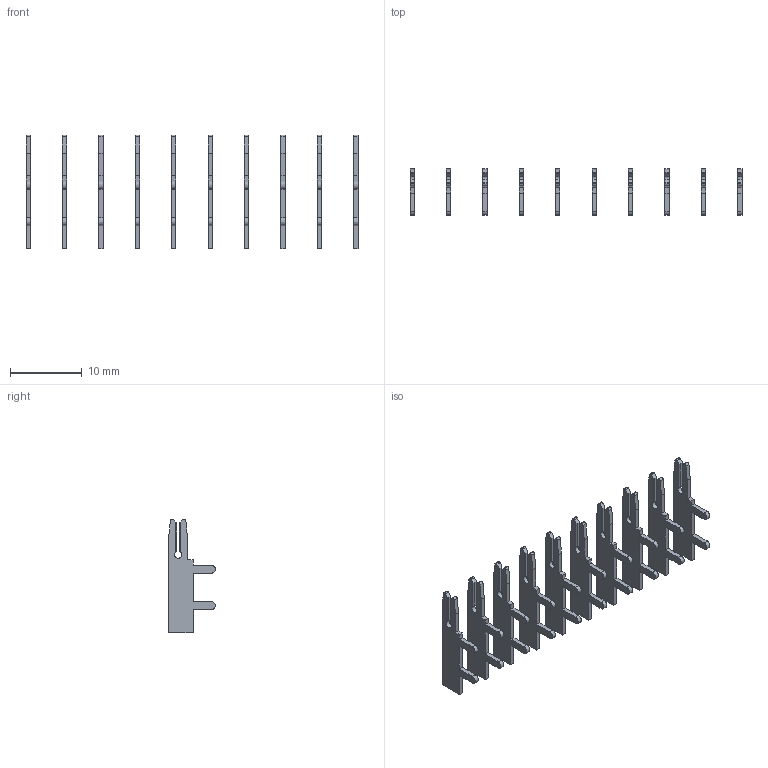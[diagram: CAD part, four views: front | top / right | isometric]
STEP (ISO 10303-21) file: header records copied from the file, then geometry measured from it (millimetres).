
FILE_DESCRIPTION (( 'STEP AP203' ), '1' );
FILE_NAME ('105-010-202-200.STEP', '2020-04-07T22:26:52', ( '' ), ( '' ), 'SwSTEP 2.0', 'SolidWorks 2016', '' );
FILE_SCHEMA (( 'CONFIG_CONTROL_DESIGN' ));
Length unit declared in the file: inch
Products named in the file (2): 105-010-202-200; 100-290-001_100-290-202
Assembly tree (10 placements, depth 2):
  105-010-202-200
    100-290-001_100-290-202  x10
Bounding box: 46.32 x 6.53 x 15.88 mm (x, y, z)
Volume: 317.7 mm3; surface area: 1413 mm2
Topology: 10 solids, 10 shells, 300 faces, 840 edges, 560 vertices
Faces by surface type: plane 230, cylinder 70
Entity records: 1450 total; most frequent: CARTESIAN_POINT 195, DIRECTION 180, ORIENTED_EDGE 168, EDGE_CURVE 84, VECTOR 66, LINE 66, AXIS2_PLACEMENT_3D 57, VERTEX_POINT 56
